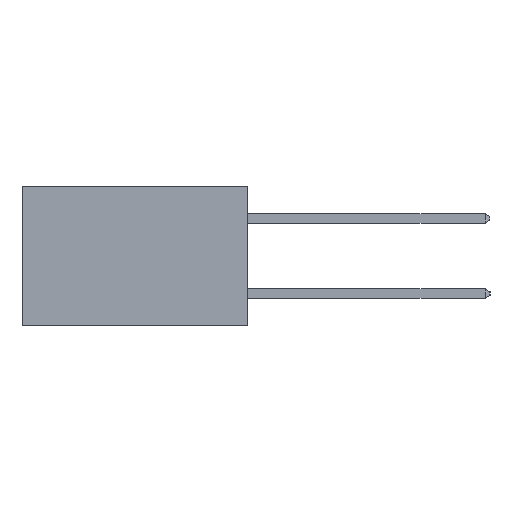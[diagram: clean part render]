
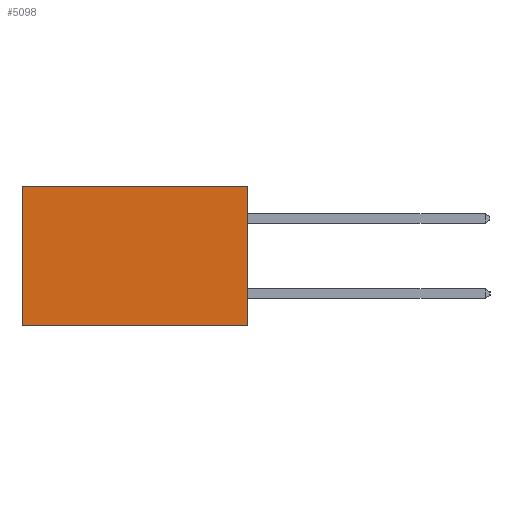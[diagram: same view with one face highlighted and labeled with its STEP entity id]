
A CAD part, left-side view. The second image highlights one B-rep face of the part: STEP entity #5098.
In plain terms, the highlighted planar face has unit normal (-1, 0, 0).
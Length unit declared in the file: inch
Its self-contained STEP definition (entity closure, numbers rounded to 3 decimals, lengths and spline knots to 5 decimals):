
#366 = CARTESIAN_POINT ( 'NONE',  ( 0.2615, 0.6, 0. ) ) ;
#397 = AXIS2_PLACEMENT_3D ( 'NONE', #1161, #1005, #978 ) ;
#415 = VECTOR ( 'NONE', #12196, 39.37008 ) ;
#597 = EDGE_CURVE ( 'NONE', #12668, #5788, #5991, .T. ) ;
#972 = EDGE_CURVE ( 'NONE', #12416, #12668, #6168, .T. ) ;
#978 = DIRECTION ( 'NONE',  ( 0., 0., -1. ) ) ;
#1005 = DIRECTION ( 'NONE',  ( 1., 0., 0. ) ) ;
#1137 = CARTESIAN_POINT ( 'NONE',  ( 0.2615, 0., 0. ) ) ;
#1161 = CARTESIAN_POINT ( 'NONE',  ( 0.2615, 0., -0.37 ) ) ;
#1271 = VECTOR ( 'NONE', #5310, 39.37008 ) ;
#1518 = CARTESIAN_POINT ( 'NONE',  ( 0.2615, 0., -0.37 ) ) ;
#1535 = PLANE ( 'NONE',  #397 ) ;
#2135 = LINE ( 'NONE', #11043, #8549 ) ;
#2286 = DIRECTION ( 'NONE',  ( 0., 1., 0. ) ) ;
#3310 = FACE_OUTER_BOUND ( 'NONE', #6443, .T. ) ;
#3406 = VECTOR ( 'NONE', #2286, 39.37008 ) ;
#4121 = EDGE_CURVE ( 'NONE', #12416, #4807, #9382, .T. ) ;
#4454 = CARTESIAN_POINT ( 'NONE',  ( 0.2615, 0., -0.37 ) ) ;
#4807 = VERTEX_POINT ( 'NONE', #1518 ) ;
#5098 = ADVANCED_FACE ( 'NONE', ( #3310 ), #1535, .F. ) ;
#5250 = ORIENTED_EDGE ( 'NONE', *, *, #972, .T. ) ;
#5310 = DIRECTION ( 'NONE',  ( 0., 0., -1. ) ) ;
#5788 = VERTEX_POINT ( 'NONE', #8192 ) ;
#5991 = LINE ( 'NONE', #11506, #415 ) ;
#6168 = LINE ( 'NONE', #11976, #3406 ) ;
#6443 = EDGE_LOOP ( 'NONE', ( #8040, #11589, #8680, #5250 ) ) ;
#6798 = EDGE_CURVE ( 'NONE', #4807, #5788, #2135, .T. ) ;
#8040 = ORIENTED_EDGE ( 'NONE', *, *, #597, .T. ) ;
#8192 = CARTESIAN_POINT ( 'NONE',  ( 0.2615, 0.6, -0.37 ) ) ;
#8549 = VECTOR ( 'NONE', #10990, 39.37008 ) ;
#8680 = ORIENTED_EDGE ( 'NONE', *, *, #4121, .F. ) ;
#9382 = LINE ( 'NONE', #4454, #1271 ) ;
#10990 = DIRECTION ( 'NONE',  ( 0., 1., 0. ) ) ;
#11043 = CARTESIAN_POINT ( 'NONE',  ( 0.2615, 0., -0.37 ) ) ;
#11506 = CARTESIAN_POINT ( 'NONE',  ( 0.2615, 0.6, -0.37 ) ) ;
#11589 = ORIENTED_EDGE ( 'NONE', *, *, #6798, .F. ) ;
#11976 = CARTESIAN_POINT ( 'NONE',  ( 0.2615, 0., 0. ) ) ;
#12196 = DIRECTION ( 'NONE',  ( 0., 0., -1. ) ) ;
#12416 = VERTEX_POINT ( 'NONE', #1137 ) ;
#12668 = VERTEX_POINT ( 'NONE', #366 ) ;
